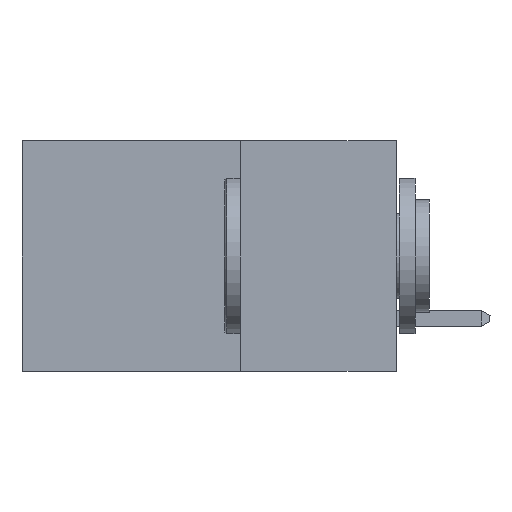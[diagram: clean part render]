
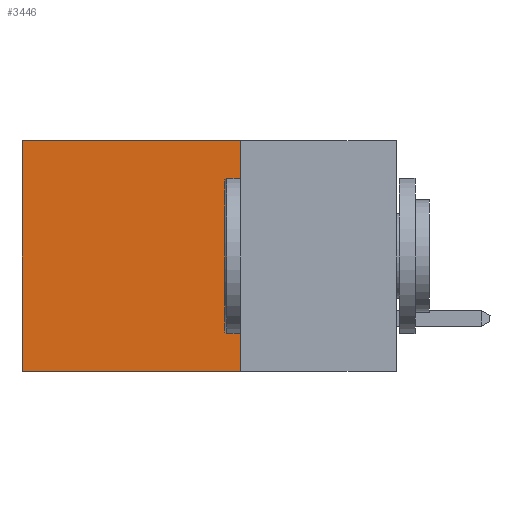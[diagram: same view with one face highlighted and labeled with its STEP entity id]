
A CAD part, left-side view. The second image highlights one B-rep face of the part: STEP entity #3446.
In plain terms, the highlighted planar face has unit normal (-1, 0, 0).
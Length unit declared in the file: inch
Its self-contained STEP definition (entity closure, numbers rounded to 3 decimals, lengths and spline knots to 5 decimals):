
#737 = CARTESIAN_POINT ( 'NONE',  ( 0.2615, 0.6, -0.37 ) ) ;
#787 = VECTOR ( 'NONE', #17395, 39.37008 ) ;
#1276 = CARTESIAN_POINT ( 'NONE',  ( 0.2615, 0.6, -0.37 ) ) ;
#1517 = CARTESIAN_POINT ( 'NONE',  ( 0.2615, 0.25, -0.37 ) ) ;
#1763 = FACE_OUTER_BOUND ( 'NONE', #5290, .T. ) ;
#1864 = CARTESIAN_POINT ( 'NONE',  ( 0.2615, 0.6, 0. ) ) ;
#2332 = VERTEX_POINT ( 'NONE', #1864 ) ;
#2462 = DIRECTION ( 'NONE',  ( 0., 0., -1. ) ) ;
#2580 = DIRECTION ( 'NONE',  ( 1., 0., 0. ) ) ;
#2602 = CARTESIAN_POINT ( 'NONE',  ( 0.2615, 0.25, -0.37 ) ) ;
#3041 = VERTEX_POINT ( 'NONE', #17909 ) ;
#3070 = PLANE ( 'NONE',  #12817 ) ;
#3355 = CARTESIAN_POINT ( 'NONE',  ( 0.2615, 0.25, -0.37 ) ) ;
#3446 = ADVANCED_FACE ( 'NONE', ( #1763 ), #3070, .F. ) ;
#4189 = EDGE_CURVE ( 'NONE', #3041, #2332, #14066, .T. ) ;
#4578 = DIRECTION ( 'NONE',  ( 0., 0., -1. ) ) ;
#5141 = LINE ( 'NONE', #3355, #787 ) ;
#5290 = EDGE_LOOP ( 'NONE', ( #11572, #18747, #19956, #6011 ) ) ;
#5829 = VECTOR ( 'NONE', #12741, 39.37008 ) ;
#6011 = ORIENTED_EDGE ( 'NONE', *, *, #4189, .T. ) ;
#6027 = CARTESIAN_POINT ( 'NONE',  ( 0.2615, 0.25, -0.37 ) ) ;
#6336 = VECTOR ( 'NONE', #7638, 39.37008 ) ;
#7090 = VERTEX_POINT ( 'NONE', #737 ) ;
#7638 = DIRECTION ( 'NONE',  ( 0., 0., -1. ) ) ;
#7680 = VERTEX_POINT ( 'NONE', #1517 ) ;
#9734 = EDGE_CURVE ( 'NONE', #2332, #7090, #14163, .T. ) ;
#11572 = ORIENTED_EDGE ( 'NONE', *, *, #9734, .T. ) ;
#12741 = DIRECTION ( 'NONE',  ( 0., 1., 0. ) ) ;
#12765 = CARTESIAN_POINT ( 'NONE',  ( 0.2615, 0.25, 0. ) ) ;
#12817 = AXIS2_PLACEMENT_3D ( 'NONE', #2602, #2580, #2462 ) ;
#13999 = EDGE_CURVE ( 'NONE', #7680, #7090, #5141, .T. ) ;
#14066 = LINE ( 'NONE', #12765, #5829 ) ;
#14163 = LINE ( 'NONE', #1276, #17741 ) ;
#17012 = EDGE_CURVE ( 'NONE', #3041, #7680, #18570, .T. ) ;
#17395 = DIRECTION ( 'NONE',  ( 0., 1., 0. ) ) ;
#17741 = VECTOR ( 'NONE', #4578, 39.37008 ) ;
#17909 = CARTESIAN_POINT ( 'NONE',  ( 0.2615, 0.25, 0. ) ) ;
#18570 = LINE ( 'NONE', #6027, #6336 ) ;
#18747 = ORIENTED_EDGE ( 'NONE', *, *, #13999, .F. ) ;
#19956 = ORIENTED_EDGE ( 'NONE', *, *, #17012, .F. ) ;
